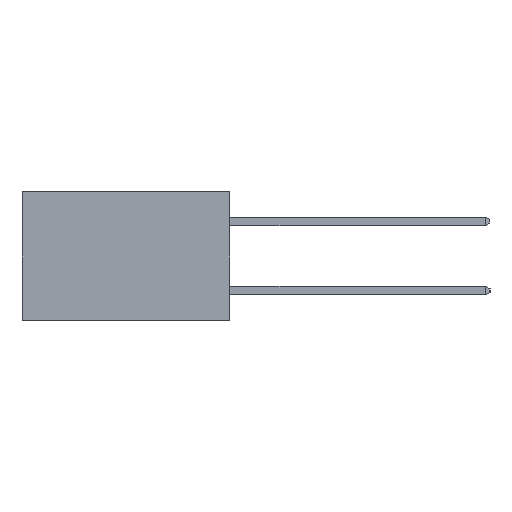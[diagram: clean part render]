
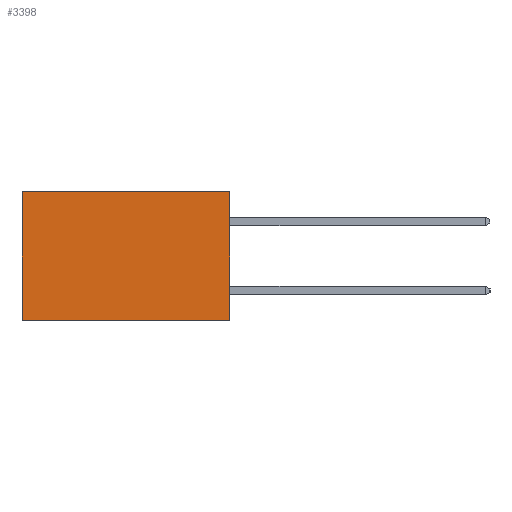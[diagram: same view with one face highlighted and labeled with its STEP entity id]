
A CAD part, left-side view. The second image highlights one B-rep face of the part: STEP entity #3398.
In plain terms, the highlighted planar face has unit normal (-1, 0, 0).
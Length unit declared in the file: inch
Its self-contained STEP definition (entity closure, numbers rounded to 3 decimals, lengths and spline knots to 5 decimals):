
#143 = CARTESIAN_POINT ( 'NONE',  ( 0.2615, 0., -0.37 ) ) ;
#163 = VERTEX_POINT ( 'NONE', #1161 ) ;
#292 = LINE ( 'NONE', #17707, #807 ) ;
#480 = FACE_OUTER_BOUND ( 'NONE', #16126, .T. ) ;
#616 = CARTESIAN_POINT ( 'NONE',  ( 0.2615, 0., 0. ) ) ;
#683 = EDGE_CURVE ( 'NONE', #16345, #163, #12982, .T. ) ;
#807 = VECTOR ( 'NONE', #7615, 39.37008 ) ;
#897 = AXIS2_PLACEMENT_3D ( 'NONE', #143, #19208, #19163 ) ;
#1161 = CARTESIAN_POINT ( 'NONE',  ( 0.2615, 0.6, -0.37 ) ) ;
#1196 = EDGE_CURVE ( 'NONE', #13254, #7390, #292, .T. ) ;
#1319 = VECTOR ( 'NONE', #9665, 39.37008 ) ;
#2639 = ORIENTED_EDGE ( 'NONE', *, *, #4897, .F. ) ;
#2641 = LINE ( 'NONE', #19319, #14649 ) ;
#3182 = ORIENTED_EDGE ( 'NONE', *, *, #1196, .F. ) ;
#3398 = ADVANCED_FACE ( 'NONE', ( #480 ), #19212, .F. ) ;
#4897 = EDGE_CURVE ( 'NONE', #7390, #163, #2641, .T. ) ;
#5038 = EDGE_CURVE ( 'NONE', #13254, #16345, #7904, .T. ) ;
#6110 = ORIENTED_EDGE ( 'NONE', *, *, #683, .T. ) ;
#7390 = VERTEX_POINT ( 'NONE', #13145 ) ;
#7615 = DIRECTION ( 'NONE',  ( 0., 0., -1. ) ) ;
#7904 = LINE ( 'NONE', #15334, #18709 ) ;
#9665 = DIRECTION ( 'NONE',  ( 0., 0., -1. ) ) ;
#12101 = DIRECTION ( 'NONE',  ( 0., 1., 0. ) ) ;
#12982 = LINE ( 'NONE', #19308, #1319 ) ;
#13145 = CARTESIAN_POINT ( 'NONE',  ( 0.2615, 0., -0.37 ) ) ;
#13254 = VERTEX_POINT ( 'NONE', #616 ) ;
#14649 = VECTOR ( 'NONE', #12101, 39.37008 ) ;
#15334 = CARTESIAN_POINT ( 'NONE',  ( 0.2615, 0., 0. ) ) ;
#16126 = EDGE_LOOP ( 'NONE', ( #6110, #2639, #3182, #19103 ) ) ;
#16345 = VERTEX_POINT ( 'NONE', #17263 ) ;
#17263 = CARTESIAN_POINT ( 'NONE',  ( 0.2615, 0.6, 0. ) ) ;
#17707 = CARTESIAN_POINT ( 'NONE',  ( 0.2615, 0., -0.37 ) ) ;
#18197 = DIRECTION ( 'NONE',  ( 0., 1., 0. ) ) ;
#18709 = VECTOR ( 'NONE', #18197, 39.37008 ) ;
#19103 = ORIENTED_EDGE ( 'NONE', *, *, #5038, .T. ) ;
#19163 = DIRECTION ( 'NONE',  ( 0., 0., -1. ) ) ;
#19208 = DIRECTION ( 'NONE',  ( 1., 0., 0. ) ) ;
#19212 = PLANE ( 'NONE',  #897 ) ;
#19308 = CARTESIAN_POINT ( 'NONE',  ( 0.2615, 0.6, -0.37 ) ) ;
#19319 = CARTESIAN_POINT ( 'NONE',  ( 0.2615, 0., -0.37 ) ) ;
